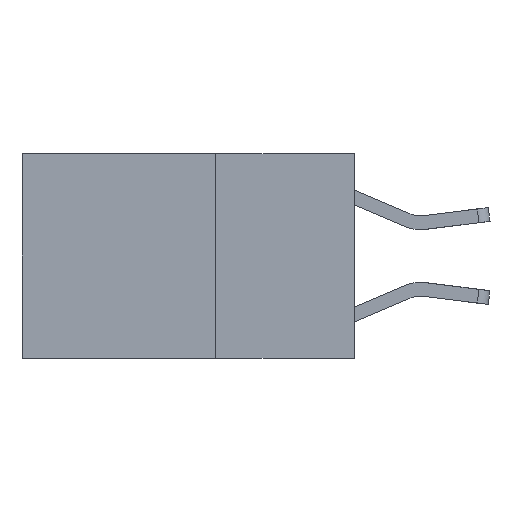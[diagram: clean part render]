
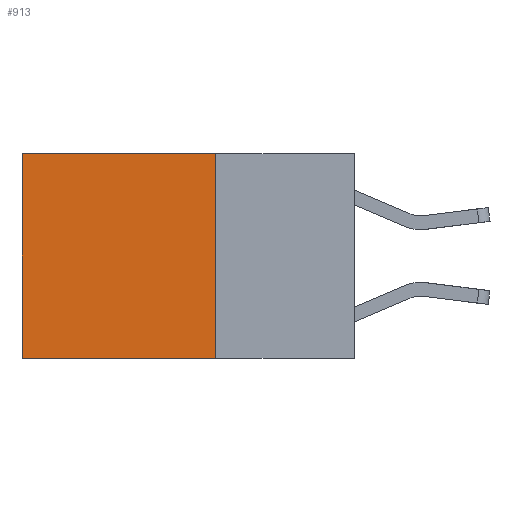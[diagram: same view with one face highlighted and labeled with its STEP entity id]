
A CAD part, left-side view. The second image highlights one B-rep face of the part: STEP entity #913.
In plain terms, the highlighted planar face has unit normal (-1, 0, 0).
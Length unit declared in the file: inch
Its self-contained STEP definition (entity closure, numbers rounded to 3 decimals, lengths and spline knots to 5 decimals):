
#469 = VERTEX_POINT ( 'NONE', #6069 ) ;
#657 = CARTESIAN_POINT ( 'NONE',  ( 0.2625, 0.25, 0. ) ) ;
#703 = LINE ( 'NONE', #9375, #10136 ) ;
#887 = EDGE_CURVE ( 'NONE', #5484, #9075, #1932, .T. ) ;
#913 = ADVANCED_FACE ( 'NONE', ( #5011 ), #3679, .F. ) ;
#1018 = EDGE_CURVE ( 'NONE', #5484, #5940, #3292, .T. ) ;
#1182 = VECTOR ( 'NONE', #6913, 39.37008 ) ;
#1337 = DIRECTION ( 'NONE',  ( 0., 0., -1. ) ) ;
#1439 = VECTOR ( 'NONE', #8394, 39.37008 ) ;
#1783 = EDGE_CURVE ( 'NONE', #5940, #469, #703, .T. ) ;
#1932 = LINE ( 'NONE', #5242, #1439 ) ;
#2201 = DIRECTION ( 'NONE',  ( 0., 0., -1. ) ) ;
#3088 = DIRECTION ( 'NONE',  ( 0., 1., 0. ) ) ;
#3097 = CARTESIAN_POINT ( 'NONE',  ( 0.2625, 0.25, -0.37 ) ) ;
#3292 = LINE ( 'NONE', #657, #8917 ) ;
#3422 = ORIENTED_EDGE ( 'NONE', *, *, #1783, .F. ) ;
#3679 = PLANE ( 'NONE',  #5938 ) ;
#4463 = ORIENTED_EDGE ( 'NONE', *, *, #9849, .T. ) ;
#4808 = CARTESIAN_POINT ( 'NONE',  ( 0.2625, 0.25, 0. ) ) ;
#5011 = FACE_OUTER_BOUND ( 'NONE', #7010, .T. ) ;
#5076 = CARTESIAN_POINT ( 'NONE',  ( 0.2625, 0.6, 0. ) ) ;
#5181 = CARTESIAN_POINT ( 'NONE',  ( 0.2625, 0.25, 0. ) ) ;
#5242 = CARTESIAN_POINT ( 'NONE',  ( 0.2625, 0.25, 0. ) ) ;
#5484 = VERTEX_POINT ( 'NONE', #4808 ) ;
#5513 = ORIENTED_EDGE ( 'NONE', *, *, #887, .T. ) ;
#5938 = AXIS2_PLACEMENT_3D ( 'NONE', #5181, #9965, #1337 ) ;
#5940 = VERTEX_POINT ( 'NONE', #3097 ) ;
#6069 = CARTESIAN_POINT ( 'NONE',  ( 0.2625, 0.6, -0.37 ) ) ;
#6162 = CARTESIAN_POINT ( 'NONE',  ( 0.2625, 0.6, 0. ) ) ;
#6913 = DIRECTION ( 'NONE',  ( 0., 0., -1. ) ) ;
#7010 = EDGE_LOOP ( 'NONE', ( #4463, #3422, #9579, #5513 ) ) ;
#8394 = DIRECTION ( 'NONE',  ( 0., 1., 0. ) ) ;
#8917 = VECTOR ( 'NONE', #2201, 39.37008 ) ;
#9075 = VERTEX_POINT ( 'NONE', #5076 ) ;
#9375 = CARTESIAN_POINT ( 'NONE',  ( 0.2625, 0.25, -0.37 ) ) ;
#9579 = ORIENTED_EDGE ( 'NONE', *, *, #1018, .F. ) ;
#9627 = LINE ( 'NONE', #6162, #1182 ) ;
#9849 = EDGE_CURVE ( 'NONE', #9075, #469, #9627, .T. ) ;
#9965 = DIRECTION ( 'NONE',  ( 1., 0., 0. ) ) ;
#10136 = VECTOR ( 'NONE', #3088, 39.37008 ) ;
